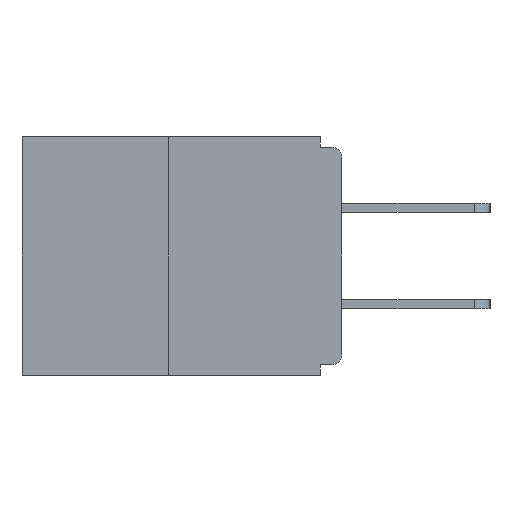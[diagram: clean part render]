
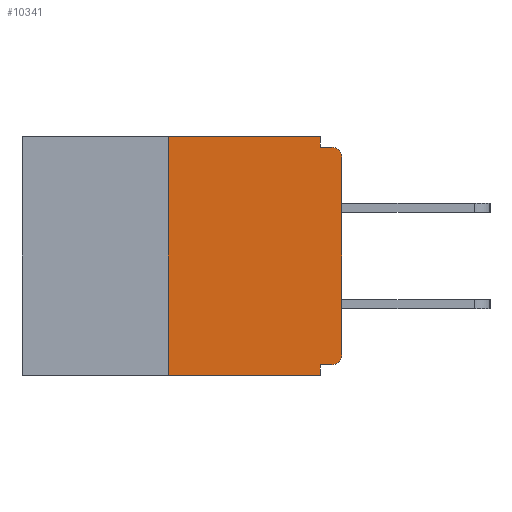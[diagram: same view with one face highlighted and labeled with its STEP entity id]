
A CAD part, left-side view. The second image highlights one B-rep face of the part: STEP entity #10341.
In plain terms, the highlighted planar face has unit normal (-1, 0, 0).
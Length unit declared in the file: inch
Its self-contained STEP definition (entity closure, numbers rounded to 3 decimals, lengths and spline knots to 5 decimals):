
#315 = EDGE_CURVE ( 'NONE', #3959, #8769, #14079, .T. ) ;
#410 = DIRECTION ( 'NONE',  ( 1., 0., 0. ) ) ;
#471 = CIRCLE ( 'NONE', #21775, 0.015 ) ;
#764 = DIRECTION ( 'NONE',  ( -1., 0., 0. ) ) ;
#795 = DIRECTION ( 'NONE',  ( 0., 1., 0. ) ) ;
#947 = EDGE_CURVE ( 'NONE', #9269, #15855, #3969, .T. ) ;
#1263 = DIRECTION ( 'NONE',  ( 0., -1., 0. ) ) ;
#1402 = AXIS2_PLACEMENT_3D ( 'NONE', #10834, #410, #21093 ) ;
#1523 = EDGE_CURVE ( 'NONE', #18879, #3537, #2815, .T. ) ;
#1806 = CARTESIAN_POINT ( 'NONE',  ( 0., 0.46, 0. ) ) ;
#2434 = CARTESIAN_POINT ( 'NONE',  ( 0., 0.031, -0.328 ) ) ;
#2649 = VECTOR ( 'NONE', #1263, 39.37008 ) ;
#2815 = LINE ( 'NONE', #14581, #9083 ) ;
#2835 = CARTESIAN_POINT ( 'NONE',  ( 0., 0.031, -0.015 ) ) ;
#2932 = EDGE_CURVE ( 'NONE', #11341, #3959, #8154, .T. ) ;
#3190 = ORIENTED_EDGE ( 'NONE', *, *, #947, .F. ) ;
#3537 = VERTEX_POINT ( 'NONE', #16857 ) ;
#3959 = VERTEX_POINT ( 'NONE', #2434 ) ;
#3969 = LINE ( 'NONE', #1806, #21918 ) ;
#4173 = EDGE_CURVE ( 'NONE', #14197, #8769, #4582, .T. ) ;
#4582 = LINE ( 'NONE', #22085, #2649 ) ;
#5173 = ORIENTED_EDGE ( 'NONE', *, *, #9385, .T. ) ;
#5361 = CARTESIAN_POINT ( 'NONE',  ( 0., 0.015, -0.328 ) ) ;
#5480 = LINE ( 'NONE', #21060, #19408 ) ;
#5842 = VECTOR ( 'NONE', #19625, 39.37008 ) ;
#5945 = ORIENTED_EDGE ( 'NONE', *, *, #1523, .F. ) ;
#5948 = CARTESIAN_POINT ( 'NONE',  ( 0., 0., -0.03 ) ) ;
#6091 = CARTESIAN_POINT ( 'NONE',  ( 0., 0.015, -0.313 ) ) ;
#6556 = EDGE_CURVE ( 'NONE', #11341, #7606, #7699, .T. ) ;
#7606 = VERTEX_POINT ( 'NONE', #18336 ) ;
#7607 = ORIENTED_EDGE ( 'NONE', *, *, #16418, .F. ) ;
#7699 = CIRCLE ( 'NONE', #22303, 0.015 ) ;
#7908 = CARTESIAN_POINT ( 'NONE',  ( 0., 0., -0.328 ) ) ;
#8005 = ORIENTED_EDGE ( 'NONE', *, *, #4173, .T. ) ;
#8154 = LINE ( 'NONE', #7908, #18748 ) ;
#8545 = CARTESIAN_POINT ( 'NONE',  ( 0., 0.25, 0. ) ) ;
#8681 = ORIENTED_EDGE ( 'NONE', *, *, #17881, .T. ) ;
#8769 = VERTEX_POINT ( 'NONE', #14596 ) ;
#9083 = VECTOR ( 'NONE', #19970, 39.37008 ) ;
#9269 = VERTEX_POINT ( 'NONE', #8545 ) ;
#9385 = EDGE_CURVE ( 'NONE', #19941, #3537, #471, .T. ) ;
#9538 = DIRECTION ( 'NONE',  ( 0., 0., -1. ) ) ;
#10099 = DIRECTION ( 'NONE',  ( 0., 0., -1. ) ) ;
#10341 = ADVANCED_FACE ( 'NONE', ( #16753 ), #10761, .F. ) ;
#10761 = PLANE ( 'NONE',  #1402 ) ;
#10834 = CARTESIAN_POINT ( 'NONE',  ( 0., 0.46, 0. ) ) ;
#11050 = CARTESIAN_POINT ( 'NONE',  ( 0., 0.031, 0. ) ) ;
#11336 = ORIENTED_EDGE ( 'NONE', *, *, #6556, .T. ) ;
#11341 = VERTEX_POINT ( 'NONE', #5361 ) ;
#11477 = CARTESIAN_POINT ( 'NONE',  ( 0., 0.031, -0.343 ) ) ;
#11744 = CARTESIAN_POINT ( 'NONE',  ( 0., 0., 0. ) ) ;
#11877 = VECTOR ( 'NONE', #10099, 39.37008 ) ;
#12565 = LINE ( 'NONE', #11744, #16908 ) ;
#13618 = ORIENTED_EDGE ( 'NONE', *, *, #14760, .F. ) ;
#13834 = DIRECTION ( 'NONE',  ( 0., 0., 1. ) ) ;
#14079 = LINE ( 'NONE', #11477, #11877 ) ;
#14197 = VERTEX_POINT ( 'NONE', #20588 ) ;
#14537 = LINE ( 'NONE', #11050, #5842 ) ;
#14581 = CARTESIAN_POINT ( 'NONE',  ( 0., 0., -0.015 ) ) ;
#14596 = CARTESIAN_POINT ( 'NONE',  ( 0., 0.031, -0.343 ) ) ;
#14760 = EDGE_CURVE ( 'NONE', #14197, #9269, #5480, .T. ) ;
#15147 = CARTESIAN_POINT ( 'NONE',  ( 0., 0.031, 0. ) ) ;
#15855 = VERTEX_POINT ( 'NONE', #15147 ) ;
#16079 = DIRECTION ( 'NONE',  ( 0., 0., -1. ) ) ;
#16418 = EDGE_CURVE ( 'NONE', #15855, #18879, #14537, .T. ) ;
#16753 = FACE_OUTER_BOUND ( 'NONE', #16856, .T. ) ;
#16856 = EDGE_LOOP ( 'NONE', ( #3190, #13618, #8005, #21922, #19830, #11336, #8681, #5173, #5945, #7607 ) ) ;
#16857 = CARTESIAN_POINT ( 'NONE',  ( 0., 0.015, -0.015 ) ) ;
#16908 = VECTOR ( 'NONE', #13834, 39.37008 ) ;
#17221 = CARTESIAN_POINT ( 'NONE',  ( 0., 0.015, -0.03 ) ) ;
#17505 = DIRECTION ( 'NONE',  ( 0., 0., 1. ) ) ;
#17770 = DIRECTION ( 'NONE',  ( 0., -1., 0. ) ) ;
#17881 = EDGE_CURVE ( 'NONE', #7606, #19941, #12565, .T. ) ;
#18336 = CARTESIAN_POINT ( 'NONE',  ( 0., 0., -0.313 ) ) ;
#18748 = VECTOR ( 'NONE', #795, 39.37008 ) ;
#18879 = VERTEX_POINT ( 'NONE', #2835 ) ;
#18952 = DIRECTION ( 'NONE',  ( -1., 0., 0. ) ) ;
#19408 = VECTOR ( 'NONE', #17505, 39.37008 ) ;
#19625 = DIRECTION ( 'NONE',  ( 0., 0., -1. ) ) ;
#19830 = ORIENTED_EDGE ( 'NONE', *, *, #2932, .F. ) ;
#19941 = VERTEX_POINT ( 'NONE', #5948 ) ;
#19970 = DIRECTION ( 'NONE',  ( 0., -1., 0. ) ) ;
#20588 = CARTESIAN_POINT ( 'NONE',  ( 0., 0.25, -0.343 ) ) ;
#21060 = CARTESIAN_POINT ( 'NONE',  ( 0., 0.25, 0. ) ) ;
#21093 = DIRECTION ( 'NONE',  ( 0., 0., -1. ) ) ;
#21775 = AXIS2_PLACEMENT_3D ( 'NONE', #17221, #18952, #16079 ) ;
#21918 = VECTOR ( 'NONE', #17770, 39.37008 ) ;
#21922 = ORIENTED_EDGE ( 'NONE', *, *, #315, .F. ) ;
#22085 = CARTESIAN_POINT ( 'NONE',  ( 0., 0.46, -0.343 ) ) ;
#22303 = AXIS2_PLACEMENT_3D ( 'NONE', #6091, #764, #9538 ) ;
